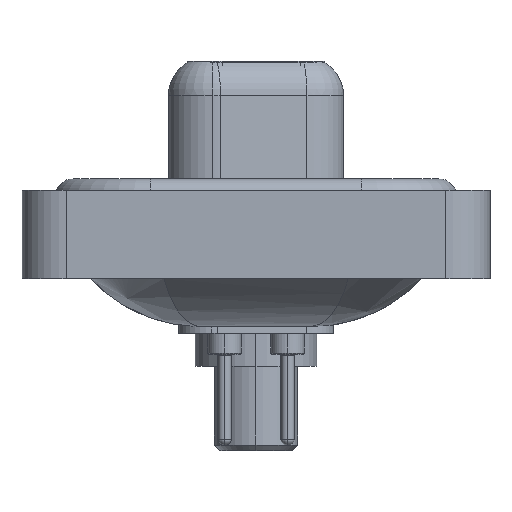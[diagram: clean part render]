
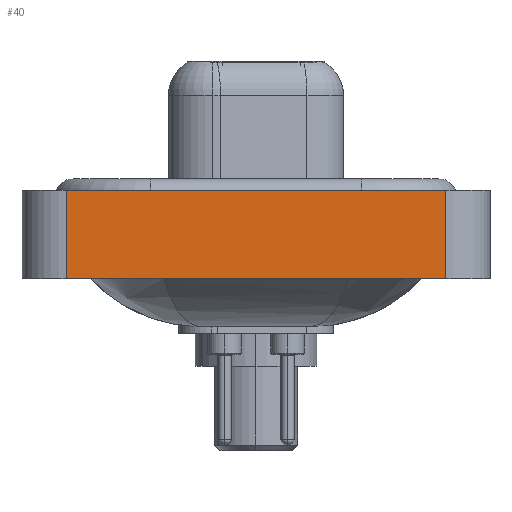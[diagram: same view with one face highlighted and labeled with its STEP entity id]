
A CAD part, left-side view. The second image highlights one B-rep face of the part: STEP entity #40.
In plain terms, the highlighted planar face has unit normal (-1, 0, 0).
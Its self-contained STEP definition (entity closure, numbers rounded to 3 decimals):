
#40 = ADVANCED_FACE ( 'NONE', ( #13746 ), #20530, .T. ) ;
#320 = CARTESIAN_POINT ( 'NONE',  ( -7.3, 8.55, 0.4 ) ) ;
#455 = EDGE_CURVE ( 'NONE', #6513, #19302, #19907, .T. ) ;
#582 = VECTOR ( 'NONE', #14438, 1000. ) ;
#716 = CARTESIAN_POINT ( 'NONE',  ( -7.3, -8.55, -3.6 ) ) ;
#1295 = CARTESIAN_POINT ( 'NONE',  ( -7.3, -8.55, -3.6 ) ) ;
#1920 = VECTOR ( 'NONE', #4192, 1000. ) ;
#1962 = EDGE_CURVE ( 'NONE', #6745, #19302, #3965, .T. ) ;
#1964 = CARTESIAN_POINT ( 'NONE',  ( -7.3, 8.55, -3.6 ) ) ;
#2480 = EDGE_CURVE ( 'NONE', #10772, #6513, #3829, .T. ) ;
#3829 = LINE ( 'NONE', #15771, #21873 ) ;
#3965 = LINE ( 'NONE', #716, #1920 ) ;
#4192 = DIRECTION ( 'NONE',  ( 0., 0., 1. ) ) ;
#5079 = CARTESIAN_POINT ( 'NONE',  ( -7.3, -8.55, 0.4 ) ) ;
#6424 = ORIENTED_EDGE ( 'NONE', *, *, #2480, .F. ) ;
#6481 = AXIS2_PLACEMENT_3D ( 'NONE', #12291, #12189, #18976 ) ;
#6513 = VERTEX_POINT ( 'NONE', #320 ) ;
#6745 = VERTEX_POINT ( 'NONE', #1295 ) ;
#8122 = ORIENTED_EDGE ( 'NONE', *, *, #455, .F. ) ;
#10772 = VERTEX_POINT ( 'NONE', #1964 ) ;
#10987 = LINE ( 'NONE', #16219, #582 ) ;
#11446 = DIRECTION ( 'NONE',  ( 0., -1., 0. ) ) ;
#11788 = CARTESIAN_POINT ( 'NONE',  ( -7.3, -8.55, 0.4 ) ) ;
#11845 = VECTOR ( 'NONE', #11446, 1000. ) ;
#12189 = DIRECTION ( 'NONE',  ( -1., 0., 0. ) ) ;
#12291 = CARTESIAN_POINT ( 'NONE',  ( -7.3, -8.55, -3.6 ) ) ;
#12429 = DIRECTION ( 'NONE',  ( 0., 0., 1. ) ) ;
#13746 = FACE_OUTER_BOUND ( 'NONE', #21990, .T. ) ;
#14438 = DIRECTION ( 'NONE',  ( 0., -1., 0. ) ) ;
#15771 = CARTESIAN_POINT ( 'NONE',  ( -7.3, 8.55, -3.6 ) ) ;
#16219 = CARTESIAN_POINT ( 'NONE',  ( -7.3, -8.55, -3.6 ) ) ;
#18353 = ORIENTED_EDGE ( 'NONE', *, *, #1962, .T. ) ;
#18976 = DIRECTION ( 'NONE',  ( 0., 0., 1. ) ) ;
#19302 = VERTEX_POINT ( 'NONE', #11788 ) ;
#19502 = EDGE_CURVE ( 'NONE', #10772, #6745, #10987, .T. ) ;
#19596 = ORIENTED_EDGE ( 'NONE', *, *, #19502, .T. ) ;
#19907 = LINE ( 'NONE', #5079, #11845 ) ;
#20530 = PLANE ( 'NONE',  #6481 ) ;
#21873 = VECTOR ( 'NONE', #12429, 1000. ) ;
#21990 = EDGE_LOOP ( 'NONE', ( #18353, #8122, #6424, #19596 ) ) ;
